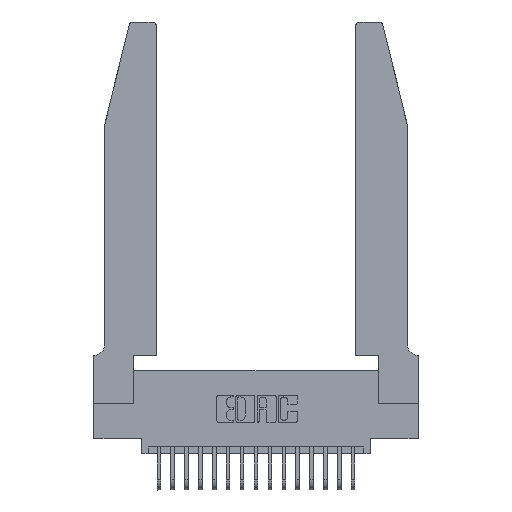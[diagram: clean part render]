
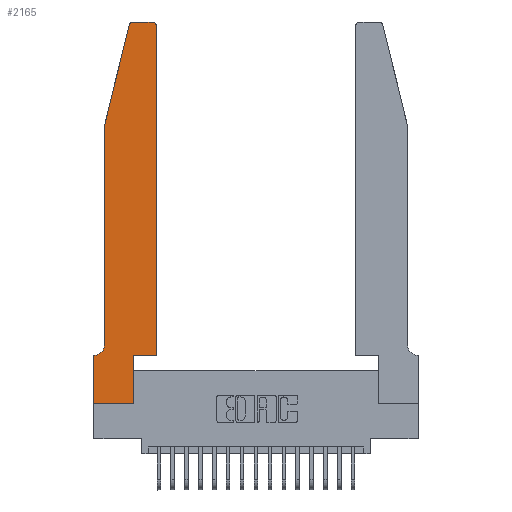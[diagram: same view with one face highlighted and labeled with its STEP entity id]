
A CAD part, top view. The second image highlights one B-rep face of the part: STEP entity #2165.
In plain terms, the highlighted planar face has unit normal (0, 0, 1).
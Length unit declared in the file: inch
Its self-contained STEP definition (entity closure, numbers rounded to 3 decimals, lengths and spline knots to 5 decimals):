
#89 = VERTEX_POINT ( 'NONE', #10615 ) ;
#328 = VERTEX_POINT ( 'NONE', #12157 ) ;
#444 = DIRECTION ( 'NONE',  ( 1., 0., 0. ) ) ;
#640 = EDGE_LOOP ( 'NONE', ( #9390, #14156, #5161, #15117, #10382, #10240, #13763, #2259, #7306, #2936, #3370, #10869 ) ) ;
#831 = LINE ( 'NONE', #12857, #16222 ) ;
#1165 = VERTEX_POINT ( 'NONE', #16046 ) ;
#1705 = CARTESIAN_POINT ( 'NONE',  ( 0.4205, 2.75, 0.37 ) ) ;
#1719 = VECTOR ( 'NONE', #6862, 39.37008 ) ;
#1724 = VERTEX_POINT ( 'NONE', #10583 ) ;
#1799 = DIRECTION ( 'NONE',  ( 1., 0., 0. ) ) ;
#1871 = DIRECTION ( 'NONE',  ( 0., 0., 1. ) ) ;
#1946 = PLANE ( 'NONE',  #4020 ) ;
#2016 = CARTESIAN_POINT ( 'NONE',  ( 0., 0.35, 0.37 ) ) ;
#2165 = ADVANCED_FACE ( 'NONE', ( #3725 ), #1946, .T. ) ;
#2259 = ORIENTED_EDGE ( 'NONE', *, *, #15589, .T. ) ;
#2318 = CARTESIAN_POINT ( 'NONE',  ( 0., 0., 0.37 ) ) ;
#2583 = CARTESIAN_POINT ( 'NONE',  ( 0.2865, 0., 0.37 ) ) ;
#2606 = CARTESIAN_POINT ( 'NONE',  ( 0.4505, 0.35, 0.37 ) ) ;
#2660 = DIRECTION ( 'NONE',  ( -1., 0., 0. ) ) ;
#2799 = VERTEX_POINT ( 'NONE', #7486 ) ;
#2936 = ORIENTED_EDGE ( 'NONE', *, *, #15040, .T. ) ;
#3349 = VERTEX_POINT ( 'NONE', #4677 ) ;
#3370 = ORIENTED_EDGE ( 'NONE', *, *, #10125, .T. ) ;
#3424 = VECTOR ( 'NONE', #5060, 39.37008 ) ;
#3530 = EDGE_CURVE ( 'NONE', #1724, #3349, #14821, .T. ) ;
#3570 = LINE ( 'NONE', #2606, #18225 ) ;
#3589 = DIRECTION ( 'NONE',  ( 0., 0., 1. ) ) ;
#3725 = FACE_OUTER_BOUND ( 'NONE', #640, .T. ) ;
#4020 = AXIS2_PLACEMENT_3D ( 'NONE', #2016, #1871, #1799 ) ;
#4130 = EDGE_CURVE ( 'NONE', #11839, #8255, #19019, .T. ) ;
#4677 = CARTESIAN_POINT ( 'NONE',  ( 0.25487, 2.72718, 0.37 ) ) ;
#5040 = LINE ( 'NONE', #18491, #9464 ) ;
#5060 = DIRECTION ( 'NONE',  ( 0., -1., 0. ) ) ;
#5161 = ORIENTED_EDGE ( 'NONE', *, *, #11949, .T. ) ;
#5934 = VERTEX_POINT ( 'NONE', #1705 ) ;
#6862 = DIRECTION ( 'NONE',  ( -0.239, -0.971, 0. ) ) ;
#6993 = LINE ( 'NONE', #15373, #14450 ) ;
#7306 = ORIENTED_EDGE ( 'NONE', *, *, #10307, .T. ) ;
#7486 = CARTESIAN_POINT ( 'NONE',  ( 0.4505, 2.72, 0.37 ) ) ;
#7909 = CARTESIAN_POINT ( 'NONE',  ( 0.0055, 0.42, 0.37 ) ) ;
#8014 = CARTESIAN_POINT ( 'NONE',  ( 0., 0., 0.37 ) ) ;
#8015 = DIRECTION ( 'NONE',  ( -1., 0., 0. ) ) ;
#8100 = DIRECTION ( 'NONE',  ( 0., 0., 1. ) ) ;
#8194 = DIRECTION ( 'NONE',  ( 1., 0., 0. ) ) ;
#8255 = VERTEX_POINT ( 'NONE', #2318 ) ;
#8256 = VECTOR ( 'NONE', #2660, 39.37008 ) ;
#8550 = EDGE_CURVE ( 'NONE', #17074, #14308, #14045, .T. ) ;
#8912 = VERTEX_POINT ( 'NONE', #2583 ) ;
#9157 = CARTESIAN_POINT ( 'NONE',  ( 0.0755, 0.42, 0.37 ) ) ;
#9382 = DIRECTION ( 'NONE',  ( -1., 0., 0. ) ) ;
#9390 = ORIENTED_EDGE ( 'NONE', *, *, #19366, .T. ) ;
#9464 = VECTOR ( 'NONE', #8015, 39.37008 ) ;
#9523 = CARTESIAN_POINT ( 'NONE',  ( 0.0055, 0.35, 0.37 ) ) ;
#9606 = CARTESIAN_POINT ( 'NONE',  ( 0.0755, 2., 0.37 ) ) ;
#9822 = CARTESIAN_POINT ( 'NONE',  ( 0.0755, 2., 0.37 ) ) ;
#10125 = EDGE_CURVE ( 'NONE', #1165, #2799, #3570, .T. ) ;
#10240 = ORIENTED_EDGE ( 'NONE', *, *, #14569, .T. ) ;
#10307 = EDGE_CURVE ( 'NONE', #8912, #89, #6993, .T. ) ;
#10382 = ORIENTED_EDGE ( 'NONE', *, *, #8550, .T. ) ;
#10449 = EDGE_CURVE ( 'NONE', #2799, #5934, #16384, .T. ) ;
#10583 = CARTESIAN_POINT ( 'NONE',  ( 0.284, 2.75, 0.37 ) ) ;
#10615 = CARTESIAN_POINT ( 'NONE',  ( 0.2865, 0.35, 0.37 ) ) ;
#10869 = ORIENTED_EDGE ( 'NONE', *, *, #10449, .T. ) ;
#11147 = DIRECTION ( 'NONE',  ( 0., -1., 0. ) ) ;
#11466 = AXIS2_PLACEMENT_3D ( 'NONE', #12685, #3589, #14168 ) ;
#11794 = DIRECTION ( 'NONE',  ( 0., 1., 0. ) ) ;
#11839 = VERTEX_POINT ( 'NONE', #15485 ) ;
#11849 = CARTESIAN_POINT ( 'NONE',  ( 0.0755, 0.35, 0.37 ) ) ;
#11949 = EDGE_CURVE ( 'NONE', #3349, #328, #17489, .T. ) ;
#12157 = CARTESIAN_POINT ( 'NONE',  ( 0.0755, 2., 0.37 ) ) ;
#12685 = CARTESIAN_POINT ( 'NONE',  ( 0.4205, 2.72, 0.37 ) ) ;
#12857 = CARTESIAN_POINT ( 'NONE',  ( 0.4505, 0.35, 0.37 ) ) ;
#13763 = ORIENTED_EDGE ( 'NONE', *, *, #4130, .T. ) ;
#14045 = CIRCLE ( 'NONE', #16729, 0.07 ) ;
#14156 = ORIENTED_EDGE ( 'NONE', *, *, #3530, .T. ) ;
#14168 = DIRECTION ( 'NONE',  ( 1., 0., 0. ) ) ;
#14248 = AXIS2_PLACEMENT_3D ( 'NONE', #17085, #8100, #18578 ) ;
#14308 = VERTEX_POINT ( 'NONE', #9523 ) ;
#14450 = VECTOR ( 'NONE', #18392, 39.37008 ) ;
#14569 = EDGE_CURVE ( 'NONE', #14308, #11839, #19271, .T. ) ;
#14821 = CIRCLE ( 'NONE', #14248, 0.03 ) ;
#15040 = EDGE_CURVE ( 'NONE', #89, #1165, #831, .T. ) ;
#15117 = ORIENTED_EDGE ( 'NONE', *, *, #19917, .T. ) ;
#15373 = CARTESIAN_POINT ( 'NONE',  ( 0.2865, 0.35, 0.37 ) ) ;
#15485 = CARTESIAN_POINT ( 'NONE',  ( 0., 0.35, 0.37 ) ) ;
#15517 = LINE ( 'NONE', #15658, #19024 ) ;
#15589 = EDGE_CURVE ( 'NONE', #8255, #8912, #15517, .T. ) ;
#15658 = CARTESIAN_POINT ( 'NONE',  ( 0., 0., 0.37 ) ) ;
#15774 = LINE ( 'NONE', #9606, #19281 ) ;
#16046 = CARTESIAN_POINT ( 'NONE',  ( 0.4505, 0.35, 0.37 ) ) ;
#16222 = VECTOR ( 'NONE', #444, 39.37008 ) ;
#16384 = CIRCLE ( 'NONE', #11466, 0.03 ) ;
#16729 = AXIS2_PLACEMENT_3D ( 'NONE', #7909, #18388, #9382 ) ;
#17074 = VERTEX_POINT ( 'NONE', #9157 ) ;
#17085 = CARTESIAN_POINT ( 'NONE',  ( 0.284, 2.72, 0.37 ) ) ;
#17489 = LINE ( 'NONE', #9822, #1719 ) ;
#18225 = VECTOR ( 'NONE', #11794, 39.37008 ) ;
#18388 = DIRECTION ( 'NONE',  ( 0., 0., -1. ) ) ;
#18392 = DIRECTION ( 'NONE',  ( 0., 1., 0. ) ) ;
#18491 = CARTESIAN_POINT ( 'NONE',  ( 0.2605, 2.75, 0.37 ) ) ;
#18578 = DIRECTION ( 'NONE',  ( 1., 0., 0. ) ) ;
#19019 = LINE ( 'NONE', #8014, #3424 ) ;
#19024 = VECTOR ( 'NONE', #8194, 39.37008 ) ;
#19271 = LINE ( 'NONE', #11849, #8256 ) ;
#19281 = VECTOR ( 'NONE', #11147, 39.37008 ) ;
#19366 = EDGE_CURVE ( 'NONE', #5934, #1724, #5040, .T. ) ;
#19917 = EDGE_CURVE ( 'NONE', #328, #17074, #15774, .T. ) ;
